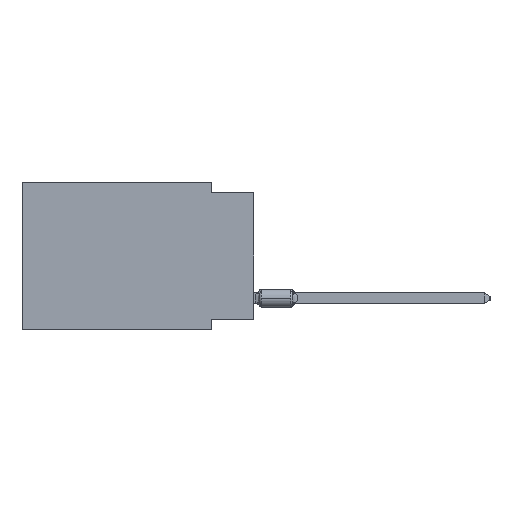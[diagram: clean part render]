
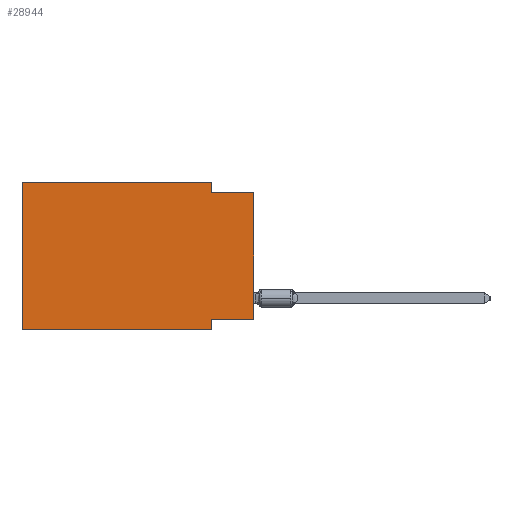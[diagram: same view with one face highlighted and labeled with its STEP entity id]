
A CAD part, left-side view. The second image highlights one B-rep face of the part: STEP entity #28944.
In plain terms, the highlighted planar face has unit normal (-1, 0, 0).
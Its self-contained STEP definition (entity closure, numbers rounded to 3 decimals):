
#111 = EDGE_CURVE ( 'NONE', #38046, #17678, #20078, .T. ) ;
#184 = DIRECTION ( 'NONE',  ( 0., 0., -1. ) ) ;
#457 = VECTOR ( 'NONE', #7827, 1000. ) ;
#743 = CARTESIAN_POINT ( 'NONE',  ( 0., 2.54, -8.89 ) ) ;
#1235 = VERTEX_POINT ( 'NONE', #4062 ) ;
#2972 = ORIENTED_EDGE ( 'NONE', *, *, #32591, .F. ) ;
#3687 = ORIENTED_EDGE ( 'NONE', *, *, #39455, .F. ) ;
#4062 = CARTESIAN_POINT ( 'NONE',  ( 0., 2.54, 0. ) ) ;
#4564 = CARTESIAN_POINT ( 'NONE',  ( 0., 2.54, 0. ) ) ;
#4749 = DIRECTION ( 'NONE',  ( 0., 0., -1. ) ) ;
#5120 = EDGE_CURVE ( 'NONE', #1235, #38736, #38051, .T. ) ;
#5312 = FACE_OUTER_BOUND ( 'NONE', #26403, .T. ) ;
#6343 = EDGE_CURVE ( 'NONE', #6989, #29412, #28317, .T. ) ;
#6989 = VERTEX_POINT ( 'NONE', #31245 ) ;
#6994 = CARTESIAN_POINT ( 'NONE',  ( 0., 0., -8.255 ) ) ;
#7414 = CARTESIAN_POINT ( 'NONE',  ( 0., 13.97, 0. ) ) ;
#7562 = EDGE_CURVE ( 'NONE', #30849, #29412, #21480, .T. ) ;
#7769 = CARTESIAN_POINT ( 'NONE',  ( 0., 0., -0.635 ) ) ;
#7827 = DIRECTION ( 'NONE',  ( 0., -1., 0. ) ) ;
#8120 = ORIENTED_EDGE ( 'NONE', *, *, #6343, .T. ) ;
#8404 = PLANE ( 'NONE',  #42025 ) ;
#9292 = CARTESIAN_POINT ( 'NONE',  ( 0., 13.97, 0. ) ) ;
#11085 = CARTESIAN_POINT ( 'NONE',  ( 0., 0., -0.635 ) ) ;
#11710 = DIRECTION ( 'NONE',  ( 0., 0., -1. ) ) ;
#11799 = CARTESIAN_POINT ( 'NONE',  ( 0., 13.97, -8.89 ) ) ;
#11980 = VERTEX_POINT ( 'NONE', #7414 ) ;
#12482 = CARTESIAN_POINT ( 'NONE',  ( 0., 13.97, 0. ) ) ;
#13031 = EDGE_CURVE ( 'NONE', #38046, #30849, #37185, .T. ) ;
#15605 = ORIENTED_EDGE ( 'NONE', *, *, #13031, .F. ) ;
#16324 = DIRECTION ( 'NONE',  ( 0., -1., 0. ) ) ;
#17241 = ORIENTED_EDGE ( 'NONE', *, *, #7562, .F. ) ;
#17678 = VERTEX_POINT ( 'NONE', #7769 ) ;
#18418 = LINE ( 'NONE', #12482, #40022 ) ;
#18518 = CARTESIAN_POINT ( 'NONE',  ( 0., 13.97, 0. ) ) ;
#19438 = DIRECTION ( 'NONE',  ( 0., 0., 1. ) ) ;
#20078 = LINE ( 'NONE', #39717, #41475 ) ;
#20412 = DIRECTION ( 'NONE',  ( 0., 1., 0. ) ) ;
#21422 = DIRECTION ( 'NONE',  ( 0., -1., 0. ) ) ;
#21480 = LINE ( 'NONE', #34940, #23033 ) ;
#22405 = CARTESIAN_POINT ( 'NONE',  ( 0., 2.54, -0.635 ) ) ;
#23033 = VECTOR ( 'NONE', #4749, 1000. ) ;
#24272 = VECTOR ( 'NONE', #20412, 1000. ) ;
#25481 = DIRECTION ( 'NONE',  ( 0., 0., 1. ) ) ;
#25493 = VECTOR ( 'NONE', #184, 1000. ) ;
#26084 = ORIENTED_EDGE ( 'NONE', *, *, #111, .T. ) ;
#26091 = VECTOR ( 'NONE', #21422, 1000. ) ;
#26403 = EDGE_LOOP ( 'NONE', ( #26084, #3687, #38519, #2972, #29767, #8120, #17241, #15605 ) ) ;
#26681 = LINE ( 'NONE', #9292, #36441 ) ;
#28317 = LINE ( 'NONE', #11799, #457 ) ;
#28944 = ADVANCED_FACE ( 'NONE', ( #5312 ), #8404, .F. ) ;
#29412 = VERTEX_POINT ( 'NONE', #743 ) ;
#29546 = DIRECTION ( 'NONE',  ( 1., 0., 0. ) ) ;
#29767 = ORIENTED_EDGE ( 'NONE', *, *, #33735, .F. ) ;
#30849 = VERTEX_POINT ( 'NONE', #35559 ) ;
#31245 = CARTESIAN_POINT ( 'NONE',  ( 0., 13.97, -8.89 ) ) ;
#32591 = EDGE_CURVE ( 'NONE', #11980, #1235, #26681, .T. ) ;
#33735 = EDGE_CURVE ( 'NONE', #6989, #11980, #18418, .T. ) ;
#34940 = CARTESIAN_POINT ( 'NONE',  ( 0., 2.54, -8.89 ) ) ;
#35559 = CARTESIAN_POINT ( 'NONE',  ( 0., 2.54, -8.255 ) ) ;
#36441 = VECTOR ( 'NONE', #16324, 1000. ) ;
#37185 = LINE ( 'NONE', #6994, #24272 ) ;
#37472 = CARTESIAN_POINT ( 'NONE',  ( 0., 0., -8.255 ) ) ;
#38046 = VERTEX_POINT ( 'NONE', #37472 ) ;
#38051 = LINE ( 'NONE', #4564, #25493 ) ;
#38519 = ORIENTED_EDGE ( 'NONE', *, *, #5120, .F. ) ;
#38736 = VERTEX_POINT ( 'NONE', #22405 ) ;
#39455 = EDGE_CURVE ( 'NONE', #38736, #17678, #41272, .T. ) ;
#39717 = CARTESIAN_POINT ( 'NONE',  ( 0., 0., 0. ) ) ;
#40022 = VECTOR ( 'NONE', #25481, 1000. ) ;
#41272 = LINE ( 'NONE', #11085, #26091 ) ;
#41475 = VECTOR ( 'NONE', #19438, 1000. ) ;
#42025 = AXIS2_PLACEMENT_3D ( 'NONE', #18518, #29546, #11710 ) ;
